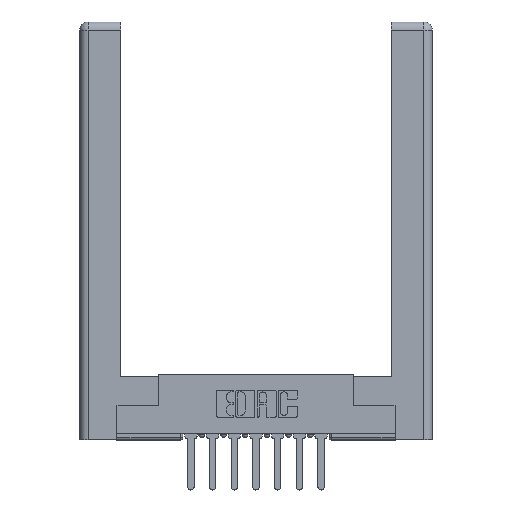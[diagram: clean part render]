
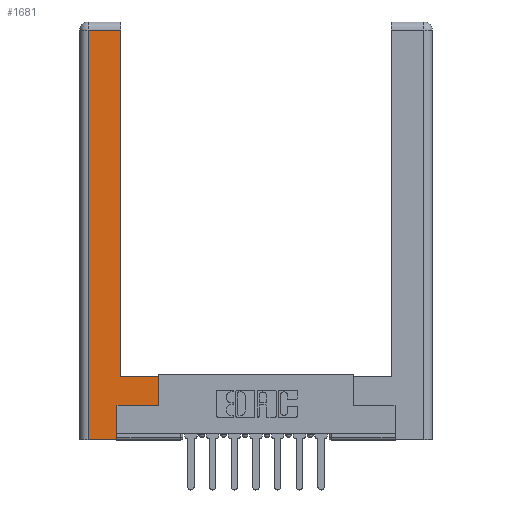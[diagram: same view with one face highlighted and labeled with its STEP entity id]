
A CAD part, top view. The second image highlights one B-rep face of the part: STEP entity #1681.
In plain terms, the highlighted planar face has unit normal (0, 0, 1).
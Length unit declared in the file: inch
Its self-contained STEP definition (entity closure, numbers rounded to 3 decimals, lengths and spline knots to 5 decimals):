
#527 = VERTEX_POINT ( 'NONE', #11104 ) ;
#715 = FACE_OUTER_BOUND ( 'NONE', #5035, .T. ) ;
#737 = CARTESIAN_POINT ( 'NONE',  ( 0.565, 0.45, 0. ) ) ;
#881 = LINE ( 'NONE', #4862, #8572 ) ;
#887 = DIRECTION ( 'NONE',  ( 1., 0., 0. ) ) ;
#998 = DIRECTION ( 'NONE',  ( 0., 1., 0. ) ) ;
#1131 = CARTESIAN_POINT ( 'NONE',  ( 0.265, 0.245, 0. ) ) ;
#1165 = VECTOR ( 'NONE', #887, 39.37008 ) ;
#1252 = LINE ( 'NONE', #3264, #6596 ) ;
#1353 = CARTESIAN_POINT ( 'NONE',  ( 0.265, 0., 0. ) ) ;
#1498 = VERTEX_POINT ( 'NONE', #11453 ) ;
#1512 = EDGE_CURVE ( 'NONE', #7863, #3982, #1252, .T. ) ;
#1541 = CARTESIAN_POINT ( 'NONE',  ( 0.0615, 0., 0. ) ) ;
#1681 = ADVANCED_FACE ( 'NONE', ( #715 ), #7657, .F. ) ;
#1747 = CARTESIAN_POINT ( 'NONE',  ( 0.565, 0.45, 0. ) ) ;
#1790 = DIRECTION ( 'NONE',  ( 0., 1., 0. ) ) ;
#2759 = LINE ( 'NONE', #5781, #5980 ) ;
#2773 = LINE ( 'NONE', #4601, #3331 ) ;
#2837 = EDGE_CURVE ( 'NONE', #1498, #7743, #881, .T. ) ;
#2890 = CARTESIAN_POINT ( 'NONE',  ( 0.295, 3., 0. ) ) ;
#3200 = EDGE_CURVE ( 'NONE', #12418, #7863, #9896, .T. ) ;
#3264 = CARTESIAN_POINT ( 'NONE',  ( 0.295, 0.45, 0. ) ) ;
#3331 = VECTOR ( 'NONE', #8598, 39.37008 ) ;
#3873 = DIRECTION ( 'NONE',  ( -1., 0., 0. ) ) ;
#3922 = EDGE_CURVE ( 'NONE', #527, #4685, #2773, .T. ) ;
#3957 = CARTESIAN_POINT ( 'NONE',  ( 0.295, 0.45, 0. ) ) ;
#3982 = VERTEX_POINT ( 'NONE', #3957 ) ;
#4566 = CARTESIAN_POINT ( 'NONE',  ( 0., 0., 0. ) ) ;
#4601 = CARTESIAN_POINT ( 'NONE',  ( 0.265, 0.245, 0. ) ) ;
#4685 = VERTEX_POINT ( 'NONE', #1131 ) ;
#4862 = CARTESIAN_POINT ( 'NONE',  ( 0.0615, 0., 0. ) ) ;
#4915 = CARTESIAN_POINT ( 'NONE',  ( 0.565, 0.245, 0. ) ) ;
#5035 = EDGE_LOOP ( 'NONE', ( #5306, #12692, #6090, #12130, #8491, #11418, #8573, #9549 ) ) ;
#5306 = ORIENTED_EDGE ( 'NONE', *, *, #5364, .T. ) ;
#5364 = EDGE_CURVE ( 'NONE', #3982, #12263, #11856, .T. ) ;
#5751 = DIRECTION ( 'NONE',  ( -1., 0., 0. ) ) ;
#5781 = CARTESIAN_POINT ( 'NONE',  ( 0.0615, 2.94, 0. ) ) ;
#5824 = DIRECTION ( 'NONE',  ( 0., 0., -1. ) ) ;
#5980 = VECTOR ( 'NONE', #3873, 39.37008 ) ;
#5997 = LINE ( 'NONE', #8865, #1165 ) ;
#6090 = ORIENTED_EDGE ( 'NONE', *, *, #2837, .T. ) ;
#6596 = VECTOR ( 'NONE', #10275, 39.37008 ) ;
#7433 = VECTOR ( 'NONE', #12340, 39.37008 ) ;
#7481 = VECTOR ( 'NONE', #998, 39.37008 ) ;
#7657 = PLANE ( 'NONE',  #9538 ) ;
#7743 = VERTEX_POINT ( 'NONE', #1541 ) ;
#7863 = VERTEX_POINT ( 'NONE', #1747 ) ;
#8155 = LINE ( 'NONE', #1353, #7433 ) ;
#8491 = ORIENTED_EDGE ( 'NONE', *, *, #3922, .T. ) ;
#8572 = VECTOR ( 'NONE', #9789, 39.37008 ) ;
#8573 = ORIENTED_EDGE ( 'NONE', *, *, #3200, .T. ) ;
#8598 = DIRECTION ( 'NONE',  ( 0., 1., 0. ) ) ;
#8865 = CARTESIAN_POINT ( 'NONE',  ( 0.565, 0.245, 0. ) ) ;
#8882 = EDGE_CURVE ( 'NONE', #7743, #527, #8155, .T. ) ;
#9111 = EDGE_CURVE ( 'NONE', #4685, #12418, #5997, .T. ) ;
#9538 = AXIS2_PLACEMENT_3D ( 'NONE', #4566, #5824, #5751 ) ;
#9549 = ORIENTED_EDGE ( 'NONE', *, *, #1512, .T. ) ;
#9789 = DIRECTION ( 'NONE',  ( 0., -1., 0. ) ) ;
#9869 = VECTOR ( 'NONE', #1790, 39.37008 ) ;
#9896 = LINE ( 'NONE', #737, #9869 ) ;
#10248 = CARTESIAN_POINT ( 'NONE',  ( 0.295, 2.94, 0. ) ) ;
#10275 = DIRECTION ( 'NONE',  ( -1., 0., 0. ) ) ;
#11104 = CARTESIAN_POINT ( 'NONE',  ( 0.265, 0., 0. ) ) ;
#11418 = ORIENTED_EDGE ( 'NONE', *, *, #9111, .T. ) ;
#11453 = CARTESIAN_POINT ( 'NONE',  ( 0.0615, 2.94, 0. ) ) ;
#11856 = LINE ( 'NONE', #2890, #7481 ) ;
#12130 = ORIENTED_EDGE ( 'NONE', *, *, #8882, .T. ) ;
#12263 = VERTEX_POINT ( 'NONE', #10248 ) ;
#12326 = EDGE_CURVE ( 'NONE', #12263, #1498, #2759, .T. ) ;
#12340 = DIRECTION ( 'NONE',  ( 1., 0., 0. ) ) ;
#12418 = VERTEX_POINT ( 'NONE', #4915 ) ;
#12692 = ORIENTED_EDGE ( 'NONE', *, *, #12326, .T. ) ;
